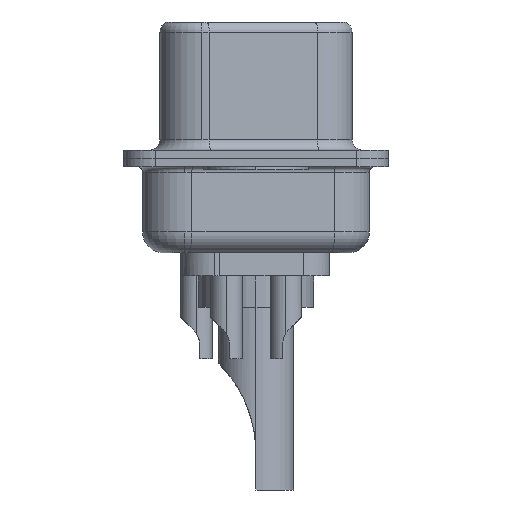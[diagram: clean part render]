
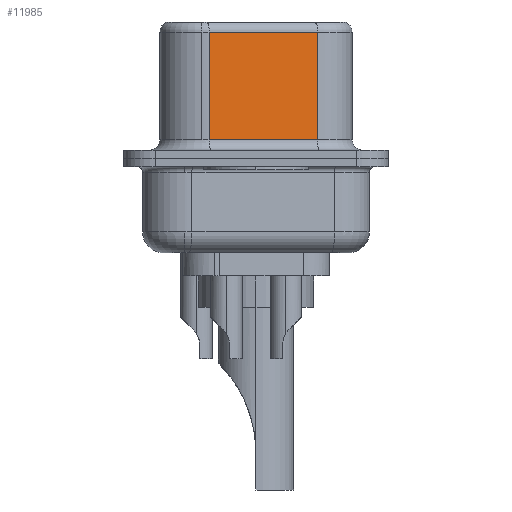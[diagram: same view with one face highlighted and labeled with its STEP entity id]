
A CAD part, left-side view. The second image highlights one B-rep face of the part: STEP entity #11985.
In plain terms, the highlighted planar face has unit normal (-0.985, -0.174, 0).
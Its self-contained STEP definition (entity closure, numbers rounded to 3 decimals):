
#1628 = DIRECTION ( 'NONE',  ( 0., 0., -1. ) ) ;
#1811 = EDGE_CURVE ( 'NONE', #14064, #8191, #8973, .T. ) ;
#2467 = ORIENTED_EDGE ( 'NONE', *, *, #1811, .F. ) ;
#2938 = CARTESIAN_POINT ( 'NONE',  ( 3.675, 2.233, 6.52 ) ) ;
#3233 = DIRECTION ( 'NONE',  ( 0., 0., -1. ) ) ;
#3375 = LINE ( 'NONE', #2938, #5881 ) ;
#3733 = DIRECTION ( 'NONE',  ( -0.174, 0.985, 0. ) ) ;
#3760 = CARTESIAN_POINT ( 'NONE',  ( 4.585, -2.927, 0.9 ) ) ;
#5070 = DIRECTION ( 'NONE',  ( -0.174, 0.985, 0. ) ) ;
#5308 = EDGE_CURVE ( 'NONE', #14640, #18486, #3375, .T. ) ;
#5721 = CARTESIAN_POINT ( 'NONE',  ( 4.585, -2.927, 0.9 ) ) ;
#5818 = CARTESIAN_POINT ( 'NONE',  ( 4.585, -2.927, 6.02 ) ) ;
#5881 = VECTOR ( 'NONE', #1628, 1000. ) ;
#6357 = VECTOR ( 'NONE', #14045, 1000. ) ;
#6533 = CARTESIAN_POINT ( 'NONE',  ( 3.675, 2.233, 6.02 ) ) ;
#6734 = PLANE ( 'NONE',  #7163 ) ;
#6933 = EDGE_CURVE ( 'NONE', #18486, #8191, #18219, .T. ) ;
#7163 = AXIS2_PLACEMENT_3D ( 'NONE', #11274, #12742, #3733 ) ;
#8191 = VERTEX_POINT ( 'NONE', #5721 ) ;
#8973 = LINE ( 'NONE', #16267, #10152 ) ;
#9306 = EDGE_LOOP ( 'NONE', ( #2467, #13687, #12386, #14452 ) ) ;
#9622 = VECTOR ( 'NONE', #5070, 1000. ) ;
#10152 = VECTOR ( 'NONE', #3233, 1000. ) ;
#11274 = CARTESIAN_POINT ( 'NONE',  ( 4.585, -2.927, 6.52 ) ) ;
#11985 = ADVANCED_FACE ( 'NONE', ( #17394 ), #6734, .F. ) ;
#12386 = ORIENTED_EDGE ( 'NONE', *, *, #5308, .T. ) ;
#12742 = DIRECTION ( 'NONE',  ( 0.985, 0.174, 0. ) ) ;
#13687 = ORIENTED_EDGE ( 'NONE', *, *, #15498, .T. ) ;
#13903 = CARTESIAN_POINT ( 'NONE',  ( 4.585, -2.927, 6.02 ) ) ;
#14045 = DIRECTION ( 'NONE',  ( 0.174, -0.985, 0. ) ) ;
#14064 = VERTEX_POINT ( 'NONE', #5818 ) ;
#14452 = ORIENTED_EDGE ( 'NONE', *, *, #6933, .T. ) ;
#14640 = VERTEX_POINT ( 'NONE', #6533 ) ;
#15498 = EDGE_CURVE ( 'NONE', #14064, #14640, #18181, .T. ) ;
#16267 = CARTESIAN_POINT ( 'NONE',  ( 4.585, -2.927, 6.52 ) ) ;
#17394 = FACE_OUTER_BOUND ( 'NONE', #9306, .T. ) ;
#18181 = LINE ( 'NONE', #13903, #9622 ) ;
#18218 = CARTESIAN_POINT ( 'NONE',  ( 3.675, 2.233, 0.9 ) ) ;
#18219 = LINE ( 'NONE', #3760, #6357 ) ;
#18486 = VERTEX_POINT ( 'NONE', #18218 ) ;
